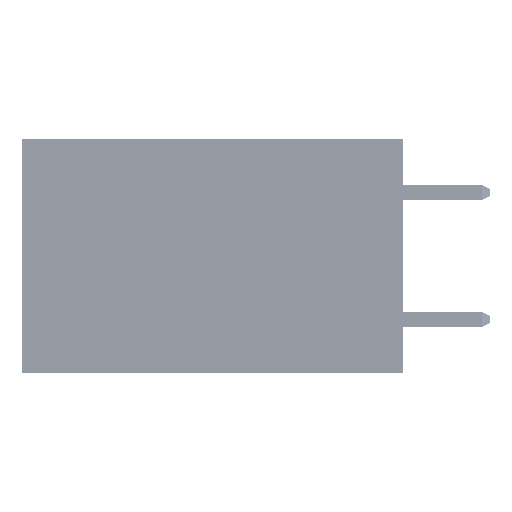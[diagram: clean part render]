
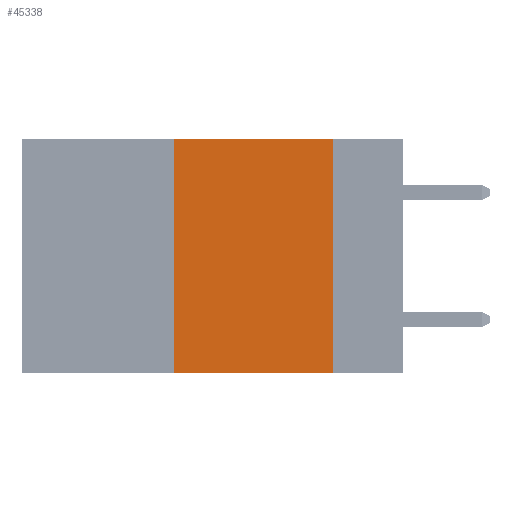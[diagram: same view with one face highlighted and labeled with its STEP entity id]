
A CAD part, left-side view. The second image highlights one B-rep face of the part: STEP entity #45338.
In plain terms, the highlighted planar face has unit normal (-1, 0, 0).
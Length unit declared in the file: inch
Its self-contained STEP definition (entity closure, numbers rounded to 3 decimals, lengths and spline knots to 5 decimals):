
#549 = VECTOR ( 'NONE', #3681, 39.37008 ) ;
#772 = ORIENTED_EDGE ( 'NONE', *, *, #18899, .F. ) ;
#1733 = ORIENTED_EDGE ( 'NONE', *, *, #3776, .F. ) ;
#1790 = DIRECTION ( 'NONE',  ( 0., 0., -1. ) ) ;
#2367 = DIRECTION ( 'NONE',  ( 0., -1., 0. ) ) ;
#3681 = DIRECTION ( 'NONE',  ( 0., -1., 0. ) ) ;
#3776 = EDGE_CURVE ( 'NONE', #30198, #10618, #37919, .T. ) ;
#3823 = DIRECTION ( 'NONE',  ( 1., 0., 0. ) ) ;
#5607 = CARTESIAN_POINT ( 'NONE',  ( 0., 0.36, 0. ) ) ;
#6135 = CARTESIAN_POINT ( 'NONE',  ( 0., 0.11, 0. ) ) ;
#6302 = VECTOR ( 'NONE', #11790, 39.37008 ) ;
#6536 = CARTESIAN_POINT ( 'NONE',  ( 0., 0.11, 0. ) ) ;
#10603 = EDGE_CURVE ( 'NONE', #20033, #51230, #32914, .T. ) ;
#10618 = VERTEX_POINT ( 'NONE', #5607 ) ;
#11217 = VECTOR ( 'NONE', #1790, 39.37008 ) ;
#11790 = DIRECTION ( 'NONE',  ( 0., 0., 1. ) ) ;
#18281 = ORIENTED_EDGE ( 'NONE', *, *, #10603, .F. ) ;
#18899 = EDGE_CURVE ( 'NONE', #10618, #20033, #46436, .T. ) ;
#19935 = CARTESIAN_POINT ( 'NONE',  ( 0., 0.6, 0. ) ) ;
#20033 = VERTEX_POINT ( 'NONE', #6536 ) ;
#21660 = AXIS2_PLACEMENT_3D ( 'NONE', #39328, #3823, #31050 ) ;
#22340 = EDGE_LOOP ( 'NONE', ( #18281, #772, #1733, #44731 ) ) ;
#23747 = EDGE_CURVE ( 'NONE', #30198, #51230, #40620, .T. ) ;
#24566 = CARTESIAN_POINT ( 'NONE',  ( 0., 0.11, -0.37 ) ) ;
#30142 = VECTOR ( 'NONE', #2367, 39.37008 ) ;
#30198 = VERTEX_POINT ( 'NONE', #30701 ) ;
#30701 = CARTESIAN_POINT ( 'NONE',  ( 0., 0.36, -0.37 ) ) ;
#30892 = PLANE ( 'NONE',  #21660 ) ;
#31050 = DIRECTION ( 'NONE',  ( 0., 0., -1. ) ) ;
#32914 = LINE ( 'NONE', #6135, #11217 ) ;
#35870 = CARTESIAN_POINT ( 'NONE',  ( 0., 0.36, 0. ) ) ;
#37919 = LINE ( 'NONE', #35870, #6302 ) ;
#39328 = CARTESIAN_POINT ( 'NONE',  ( 0., 0.6, 0. ) ) ;
#40620 = LINE ( 'NONE', #49499, #30142 ) ;
#44731 = ORIENTED_EDGE ( 'NONE', *, *, #23747, .T. ) ;
#45338 = ADVANCED_FACE ( 'NONE', ( #47943 ), #30892, .F. ) ;
#46436 = LINE ( 'NONE', #19935, #549 ) ;
#47943 = FACE_OUTER_BOUND ( 'NONE', #22340, .T. ) ;
#49499 = CARTESIAN_POINT ( 'NONE',  ( 0., 0.6, -0.37 ) ) ;
#51230 = VERTEX_POINT ( 'NONE', #24566 ) ;
